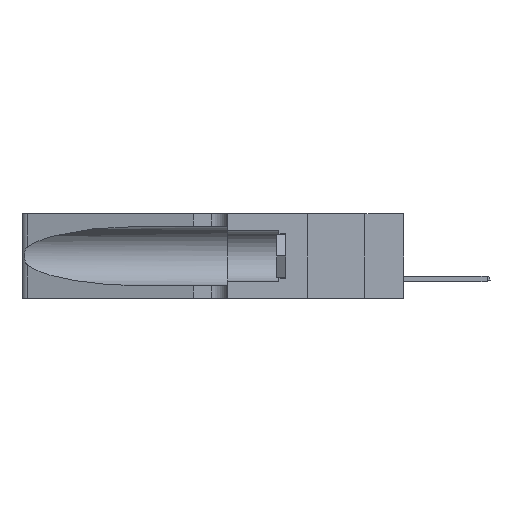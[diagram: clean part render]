
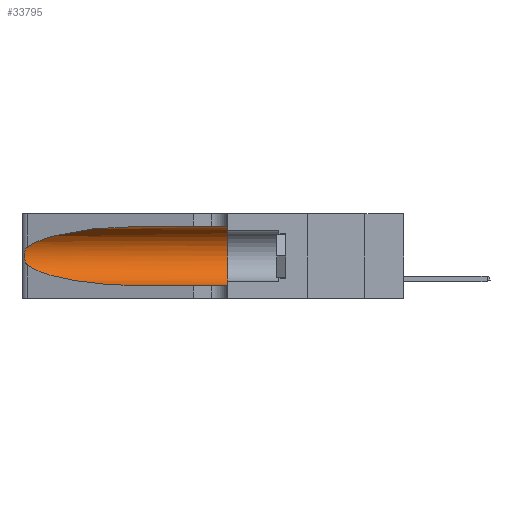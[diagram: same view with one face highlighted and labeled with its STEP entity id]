
A CAD part, left-side view. The second image highlights one B-rep face of the part: STEP entity #33795.
In plain terms, the highlighted cylindrical face has radius 3.308 mm (diameter 6.617 mm), a partial arc.
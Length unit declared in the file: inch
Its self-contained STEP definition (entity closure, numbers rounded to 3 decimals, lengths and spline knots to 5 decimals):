
#2041 = ORIENTED_EDGE ( 'NONE', *, *, #43514, .T. ) ;
#3566 = FACE_OUTER_BOUND ( 'NONE', #17889, .T. ) ;
#4947 =( BOUNDED_CURVE ( )  B_SPLINE_CURVE ( 3, ( #5561, #22945, #6960, #35150 ),
 .UNSPECIFIED., .F., .T. ) 
 B_SPLINE_CURVE_WITH_KNOTS ( ( 4, 4 ),
 ( 3.44316, 4.71239 ),
 .UNSPECIFIED. ) 
 CURVE ( )  GEOMETRIC_REPRESENTATION_ITEM ( )  RATIONAL_B_SPLINE_CURVE ( ( 1., 0.87, 0.87, 1. ) ) 
 REPRESENTATION_ITEM ( '' )  );
#5432 = LINE ( 'NONE', #6830, #32887 ) ;
#5470 = CARTESIAN_POINT ( 'NONE',  ( 0.25787, 1.23484, 0.2124 ) ) ;
#5479 = DIRECTION ( 'NONE',  ( 0., -1., 0. ) ) ;
#5561 = CARTESIAN_POINT ( 'NONE',  ( 0.25487, 1.22718, 0.14631 ) ) ;
#5617 = CARTESIAN_POINT ( 'NONE',  ( 0.26018, 1.23835, 0.19895 ) ) ;
#6575 = VERTEX_POINT ( 'NONE', #32123 ) ;
#6806 = AXIS2_PLACEMENT_3D ( 'NONE', #37369, #16256, #40883 ) ;
#6830 = CARTESIAN_POINT ( 'NONE',  ( 0.1305, 1.61858, 0.05475 ) ) ;
#6960 = CARTESIAN_POINT ( 'NONE',  ( 0.18966, 0.96281, 0.05475 ) ) ;
#7754 = EDGE_CURVE ( 'NONE', #6575, #25296, #37761, .T. ) ;
#9360 = EDGE_CURVE ( 'NONE', #11232, #23302, #5432, .T. ) ;
#10017 = ORIENTED_EDGE ( 'NONE', *, *, #15332, .F. ) ;
#11232 = VERTEX_POINT ( 'NONE', #23616 ) ;
#12913 = CARTESIAN_POINT ( 'NONE',  ( 0.26075, 1.23896, 0.178 ) ) ;
#14491 = VERTEX_POINT ( 'NONE', #22912 ) ;
#14612 = VECTOR ( 'NONE', #16751, 39.37008 ) ;
#14692 = CIRCLE ( 'NONE', #6806, 0.13025 ) ;
#15332 = EDGE_CURVE ( 'NONE', #43815, #23302, #14692, .T. ) ;
#15720 =( BOUNDED_CURVE ( )  B_SPLINE_CURVE ( 3, ( #30039, #22347, #26365, #26193 ),
 .UNSPECIFIED., .F., .F. ) 
 B_SPLINE_CURVE_WITH_KNOTS ( ( 4, 4 ),
 ( 1.5708, 2.84003 ),
 .UNSPECIFIED. ) 
 CURVE ( )  GEOMETRIC_REPRESENTATION_ITEM ( )  RATIONAL_B_SPLINE_CURVE ( ( 1., 0.87, 0.87, 1. ) ) 
 REPRESENTATION_ITEM ( '' )  );
#16256 = DIRECTION ( 'NONE',  ( 0., 1., 0. ) ) ;
#16751 = DIRECTION ( 'NONE',  ( 0., -1., 0. ) ) ;
#17889 = EDGE_LOOP ( 'NONE', ( #2041, #28336, #21113, #37448, #10017, #43796 ) ) ;
#18849 = CARTESIAN_POINT ( 'NONE',  ( 0.25487, 1.22718, 0.22369 ) ) ;
#19520 = EDGE_CURVE ( 'NONE', #25296, #11232, #4947, .T. ) ;
#21113 = ORIENTED_EDGE ( 'NONE', *, *, #19520, .T. ) ;
#22347 = CARTESIAN_POINT ( 'NONE',  ( 0.18966, 0.96281, 0.31525 ) ) ;
#22548 = CARTESIAN_POINT ( 'NONE',  ( 0.25555, 1.22994, 0.2215 ) ) ;
#22912 = CARTESIAN_POINT ( 'NONE',  ( 0.1305, 0.72297, 0.31525 ) ) ;
#22945 = CARTESIAN_POINT ( 'NONE',  ( 0.2373, 1.15595, 0.08982 ) ) ;
#23025 = CARTESIAN_POINT ( 'NONE',  ( 0.1305, 1.61858, 0.185 ) ) ;
#23302 = VERTEX_POINT ( 'NONE', #29057 ) ;
#23616 = CARTESIAN_POINT ( 'NONE',  ( 0.1305, 0.72297, 0.05475 ) ) ;
#25296 = VERTEX_POINT ( 'NONE', #42125 ) ;
#26087 = CARTESIAN_POINT ( 'NONE',  ( 0.25639, 1.23184, 0.21858 ) ) ;
#26191 = CARTESIAN_POINT ( 'NONE',  ( 0.25856, 1.23593, 0.16098 ) ) ;
#26193 = CARTESIAN_POINT ( 'NONE',  ( 0.25487, 1.22718, 0.22369 ) ) ;
#26365 = CARTESIAN_POINT ( 'NONE',  ( 0.2373, 1.15595, 0.28018 ) ) ;
#26405 = EDGE_CURVE ( 'NONE', #14491, #43815, #41074, .T. ) ;
#27150 = CARTESIAN_POINT ( 'NONE',  ( 0.25789, 1.23486, 0.15765 ) ) ;
#28040 = CARTESIAN_POINT ( 'NONE',  ( 0.1305, 0.35, 0.31525 ) ) ;
#28336 = ORIENTED_EDGE ( 'NONE', *, *, #7754, .T. ) ;
#29057 = CARTESIAN_POINT ( 'NONE',  ( 0.1305, 0.35, 0.05475 ) ) ;
#29516 = CYLINDRICAL_SURFACE ( 'NONE', #43243, 0.13025 ) ;
#29800 = DIRECTION ( 'NONE',  ( 0., 0., -1. ) ) ;
#30039 = CARTESIAN_POINT ( 'NONE',  ( 0.1305, 0.72297, 0.31525 ) ) ;
#32123 = CARTESIAN_POINT ( 'NONE',  ( 0.25487, 1.22718, 0.22369 ) ) ;
#32887 = VECTOR ( 'NONE', #41478, 39.37008 ) ;
#33795 = ADVANCED_FACE ( 'NONE', ( #3566 ), #29516, .F. ) ;
#33819 = CARTESIAN_POINT ( 'NONE',  ( 0.26075, 1.23896, 0.19203 ) ) ;
#35150 = CARTESIAN_POINT ( 'NONE',  ( 0.1305, 0.72297, 0.05475 ) ) ;
#37227 = CARTESIAN_POINT ( 'NONE',  ( 0.25639, 1.23186, 0.15144 ) ) ;
#37369 = CARTESIAN_POINT ( 'NONE',  ( 0.1305, 0.35, 0.185 ) ) ;
#37448 = ORIENTED_EDGE ( 'NONE', *, *, #9360, .T. ) ;
#37761 = B_SPLINE_CURVE_WITH_KNOTS ( 'NONE', 3,
 ( #18849, #22548, #26087, #5470, #40708, #5617, #33819, #12913, #44588, #26191, #27150, #37227, #40770, #41148 ),
 .UNSPECIFIED., .F., .F.,
 ( 4, 2, 2, 2, 2, 2, 4 ),
 ( 0., 0.00027, 0.00053, 0.00107, 0.0016, 0.00187, 0.00214 ),
 .UNSPECIFIED. ) ;
#38018 = CARTESIAN_POINT ( 'NONE',  ( 0.1305, 1.61858, 0.31525 ) ) ;
#40708 = CARTESIAN_POINT ( 'NONE',  ( 0.25854, 1.2359, 0.20912 ) ) ;
#40770 = CARTESIAN_POINT ( 'NONE',  ( 0.25555, 1.22993, 0.14849 ) ) ;
#40883 = DIRECTION ( 'NONE',  ( 0., 0., 1. ) ) ;
#41074 = LINE ( 'NONE', #38018, #14612 ) ;
#41148 = CARTESIAN_POINT ( 'NONE',  ( 0.25487, 1.22718, 0.14631 ) ) ;
#41478 = DIRECTION ( 'NONE',  ( 0., -1., 0. ) ) ;
#42125 = CARTESIAN_POINT ( 'NONE',  ( 0.25487, 1.22718, 0.14631 ) ) ;
#43243 = AXIS2_PLACEMENT_3D ( 'NONE', #23025, #5479, #29800 ) ;
#43514 = EDGE_CURVE ( 'NONE', #14491, #6575, #15720, .T. ) ;
#43796 = ORIENTED_EDGE ( 'NONE', *, *, #26405, .F. ) ;
#43815 = VERTEX_POINT ( 'NONE', #28040 ) ;
#44588 = CARTESIAN_POINT ( 'NONE',  ( 0.26017, 1.23833, 0.17102 ) ) ;
